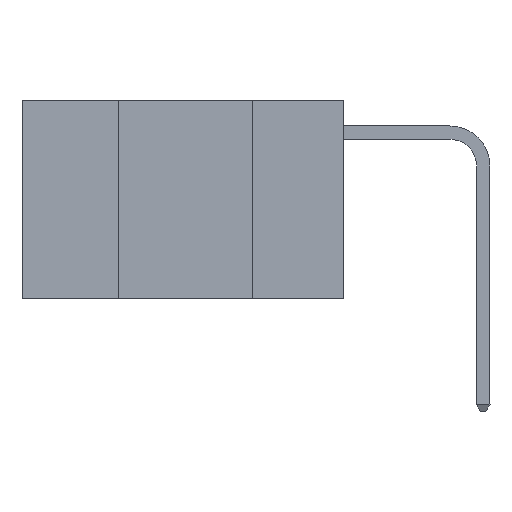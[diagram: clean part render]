
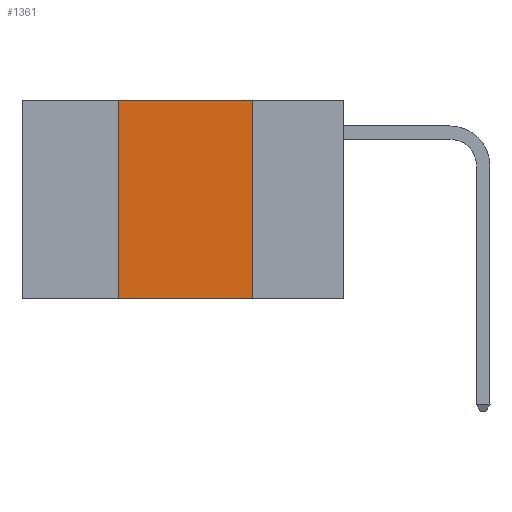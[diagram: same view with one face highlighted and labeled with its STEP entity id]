
A CAD part, left-side view. The second image highlights one B-rep face of the part: STEP entity #1361.
In plain terms, the highlighted planar face has unit normal (-1, 0, 0).
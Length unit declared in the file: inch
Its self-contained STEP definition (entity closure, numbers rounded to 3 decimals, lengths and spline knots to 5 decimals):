
#757 = DIRECTION ( 'NONE',  ( 0., 0., -1. ) ) ;
#970 = VERTEX_POINT ( 'NONE', #6770 ) ;
#1361 = ADVANCED_FACE ( 'NONE', ( #1527 ), #7739, .F. ) ;
#1527 = FACE_OUTER_BOUND ( 'NONE', #5702, .T. ) ;
#1896 = LINE ( 'NONE', #12507, #9716 ) ;
#2178 = EDGE_CURVE ( 'NONE', #12746, #2996, #9058, .T. ) ;
#2474 = CARTESIAN_POINT ( 'NONE',  ( 0., 0.42, -0.37 ) ) ;
#2996 = VERTEX_POINT ( 'NONE', #3456 ) ;
#3025 = VERTEX_POINT ( 'NONE', #2474 ) ;
#3456 = CARTESIAN_POINT ( 'NONE',  ( 0., 0.17, 0. ) ) ;
#3964 = CARTESIAN_POINT ( 'NONE',  ( 0., 0.17, 0. ) ) ;
#5702 = EDGE_LOOP ( 'NONE', ( #12675, #13252, #12685, #12422 ) ) ;
#5790 = VECTOR ( 'NONE', #757, 39.37008 ) ;
#6233 = DIRECTION ( 'NONE',  ( 0., -1., 0. ) ) ;
#6770 = CARTESIAN_POINT ( 'NONE',  ( 0., 0.17, -0.37 ) ) ;
#7329 = DIRECTION ( 'NONE',  ( 0., 0., -1. ) ) ;
#7342 = VECTOR ( 'NONE', #13093, 39.37008 ) ;
#7379 = DIRECTION ( 'NONE',  ( 1., 0., 0. ) ) ;
#7621 = CARTESIAN_POINT ( 'NONE',  ( 0., 0.6, 0. ) ) ;
#7739 = PLANE ( 'NONE',  #8284 ) ;
#7965 = LINE ( 'NONE', #3964, #5790 ) ;
#8284 = AXIS2_PLACEMENT_3D ( 'NONE', #7621, #7379, #7329 ) ;
#8685 = CARTESIAN_POINT ( 'NONE',  ( 0., 0.42, 0. ) ) ;
#9058 = LINE ( 'NONE', #12638, #11861 ) ;
#9716 = VECTOR ( 'NONE', #6233, 39.37008 ) ;
#10149 = LINE ( 'NONE', #12054, #7342 ) ;
#10341 = EDGE_CURVE ( 'NONE', #3025, #970, #1896, .T. ) ;
#11733 = EDGE_CURVE ( 'NONE', #3025, #12746, #10149, .T. ) ;
#11861 = VECTOR ( 'NONE', #12688, 39.37008 ) ;
#12054 = CARTESIAN_POINT ( 'NONE',  ( 0., 0.42, 0. ) ) ;
#12422 = ORIENTED_EDGE ( 'NONE', *, *, #10341, .T. ) ;
#12507 = CARTESIAN_POINT ( 'NONE',  ( 0., 0.6, -0.37 ) ) ;
#12638 = CARTESIAN_POINT ( 'NONE',  ( 0., 0.6, 0. ) ) ;
#12675 = ORIENTED_EDGE ( 'NONE', *, *, #13138, .F. ) ;
#12685 = ORIENTED_EDGE ( 'NONE', *, *, #11733, .F. ) ;
#12688 = DIRECTION ( 'NONE',  ( 0., -1., 0. ) ) ;
#12746 = VERTEX_POINT ( 'NONE', #8685 ) ;
#13093 = DIRECTION ( 'NONE',  ( 0., 0., 1. ) ) ;
#13138 = EDGE_CURVE ( 'NONE', #2996, #970, #7965, .T. ) ;
#13252 = ORIENTED_EDGE ( 'NONE', *, *, #2178, .F. ) ;
